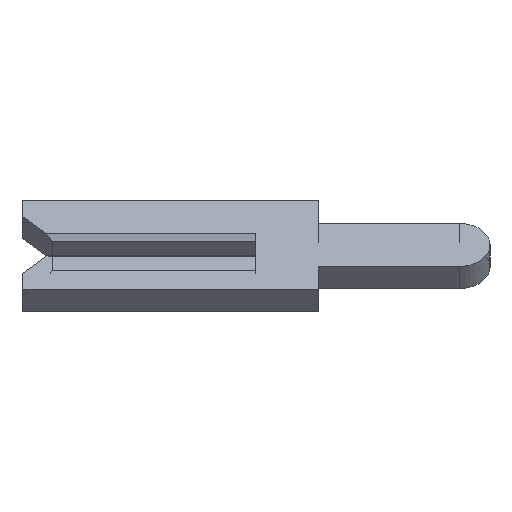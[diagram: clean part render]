
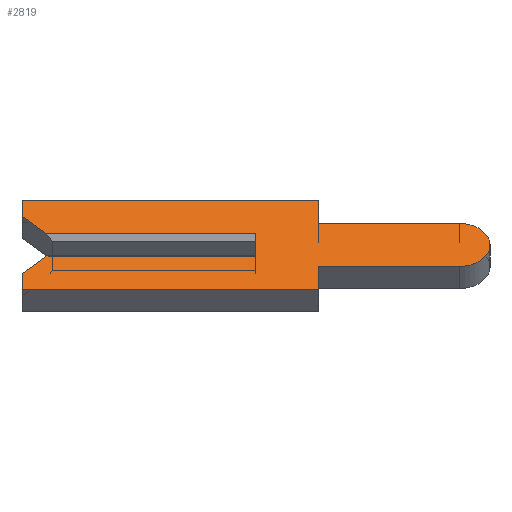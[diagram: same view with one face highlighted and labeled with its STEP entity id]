
A CAD part, left-side view. The second image highlights one B-rep face of the part: STEP entity #2819.
In plain terms, the highlighted face is planar.
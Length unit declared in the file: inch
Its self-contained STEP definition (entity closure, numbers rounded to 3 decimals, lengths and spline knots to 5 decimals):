
#10 = CARTESIAN_POINT ( 'NONE',  ( -0.01, 0.134, 0.01 ) ) ;
#25 = ORIENTED_EDGE ( 'NONE', *, *, #1651, .F. ) ;
#40 = CARTESIAN_POINT ( 'NONE',  ( -0.01, 0., -0.01 ) ) ;
#110 = CARTESIAN_POINT ( 'NONE',  ( -0.01, 0.15, 0.026 ) ) ;
#130 = CARTESIAN_POINT ( 'NONE',  ( -0.01, 0.15, -0.026 ) ) ;
#132 = FACE_OUTER_BOUND ( 'NONE', #2468, .T. ) ;
#165 = CARTESIAN_POINT ( 'NONE',  ( -0.01, 0.15, 0.01 ) ) ;
#308 = PLANE ( 'NONE',  #2267 ) ;
#331 = EDGE_CURVE ( 'NONE', #1986, #528, #2577, .T. ) ;
#369 = DIRECTION ( 'NONE',  ( 0., -1., 0. ) ) ;
#422 = VECTOR ( 'NONE', #481, 39.37008 ) ;
#441 = EDGE_CURVE ( 'NONE', #500, #1986, #459, .T. ) ;
#455 = VERTEX_POINT ( 'NONE', #2273 ) ;
#459 = LINE ( 'NONE', #110, #1696 ) ;
#465 = DIRECTION ( 'NONE',  ( 1., 0., 0. ) ) ;
#481 = DIRECTION ( 'NONE',  ( 0., 1., 0. ) ) ;
#493 = VECTOR ( 'NONE', #1460, 39.37008 ) ;
#500 = VERTEX_POINT ( 'NONE', #1653 ) ;
#506 = CARTESIAN_POINT ( 'NONE',  ( -0.01, 0.1305, -0.0065 ) ) ;
#528 = VERTEX_POINT ( 'NONE', #2779 ) ;
#538 = ORIENTED_EDGE ( 'NONE', *, *, #2256, .F. ) ;
#565 = VECTOR ( 'NONE', #2634, 39.37008 ) ;
#592 = CARTESIAN_POINT ( 'NONE',  ( -0.01, 0., 0.0065 ) ) ;
#615 = DIRECTION ( 'NONE',  ( 0., 0., -1. ) ) ;
#634 = CARTESIAN_POINT ( 'NONE',  ( -0.01, -0.04, -0.0195 ) ) ;
#653 = CARTESIAN_POINT ( 'NONE',  ( -0.01, -0.04, 0.04 ) ) ;
#698 = LINE ( 'NONE', #1627, #565 ) ;
#727 = VECTOR ( 'NONE', #1073, 39.37008 ) ;
#734 = DIRECTION ( 'NONE',  ( 0., 0., 1. ) ) ;
#789 = CARTESIAN_POINT ( 'NONE',  ( -0.01, 0., 0.01 ) ) ;
#831 = LINE ( 'NONE', #506, #1555 ) ;
#937 = VERTEX_POINT ( 'NONE', #1872 ) ;
#1053 = VECTOR ( 'NONE', #1466, 39.37008 ) ;
#1072 = EDGE_CURVE ( 'NONE', #937, #2539, #1992, .T. ) ;
#1073 = DIRECTION ( 'NONE',  ( 0., 1., 0. ) ) ;
#1092 = CARTESIAN_POINT ( 'NONE',  ( -0.01, 0.134, -0.01 ) ) ;
#1100 = CIRCLE ( 'NONE', #1520, 0.0195 ) ;
#1109 = VERTEX_POINT ( 'NONE', #2127 ) ;
#1183 = ORIENTED_EDGE ( 'NONE', *, *, #441, .F. ) ;
#1185 = CARTESIAN_POINT ( 'NONE',  ( -0.01, -0.1305, -0.0195 ) ) ;
#1255 = EDGE_CURVE ( 'NONE', #2694, #1566, #1958, .T. ) ;
#1326 = ORIENTED_EDGE ( 'NONE', *, *, #1428, .T. ) ;
#1346 = VECTOR ( 'NONE', #1954, 39.37008 ) ;
#1360 = EDGE_CURVE ( 'NONE', #1774, #2841, #2565, .T. ) ;
#1376 = DIRECTION ( 'NONE',  ( 0., -0.707, 0.707 ) ) ;
#1396 = CARTESIAN_POINT ( 'NONE',  ( -0.01, 0.15, -0.026 ) ) ;
#1405 = VECTOR ( 'NONE', #2118, 39.37008 ) ;
#1410 = DIRECTION ( 'NONE',  ( 0., 0., -1. ) ) ;
#1428 = EDGE_CURVE ( 'NONE', #2333, #1566, #2649, .T. ) ;
#1459 = LINE ( 'NONE', #1759, #1346 ) ;
#1460 = DIRECTION ( 'NONE',  ( 0., -1., 0. ) ) ;
#1466 = DIRECTION ( 'NONE',  ( 0., 0., 1. ) ) ;
#1472 = CARTESIAN_POINT ( 'NONE',  ( -0.01, -0.04, -0.04 ) ) ;
#1488 = LINE ( 'NONE', #1965, #2746 ) ;
#1520 = AXIS2_PLACEMENT_3D ( 'NONE', #2249, #465, #2211 ) ;
#1538 = DIRECTION ( 'NONE',  ( 0., 0., -1. ) ) ;
#1555 = VECTOR ( 'NONE', #1376, 39.37008 ) ;
#1566 = VERTEX_POINT ( 'NONE', #789 ) ;
#1579 = VECTOR ( 'NONE', #615, 39.37008 ) ;
#1627 = CARTESIAN_POINT ( 'NONE',  ( -0.01, 0.1305, 0.0065 ) ) ;
#1633 = ORIENTED_EDGE ( 'NONE', *, *, #1360, .F. ) ;
#1651 = EDGE_CURVE ( 'NONE', #2333, #500, #698, .T. ) ;
#1653 = CARTESIAN_POINT ( 'NONE',  ( -0.01, 0.15, 0.026 ) ) ;
#1696 = VECTOR ( 'NONE', #734, 39.37008 ) ;
#1700 = VERTEX_POINT ( 'NONE', #1092 ) ;
#1706 = EDGE_CURVE ( 'NONE', #1700, #2694, #1488, .T. ) ;
#1758 = EDGE_CURVE ( 'NONE', #2799, #1774, #2646, .T. ) ;
#1759 = CARTESIAN_POINT ( 'NONE',  ( -0.01, -0.04, 0.0195 ) ) ;
#1767 = ORIENTED_EDGE ( 'NONE', *, *, #1706, .F. ) ;
#1774 = VERTEX_POINT ( 'NONE', #2425 ) ;
#1799 = EDGE_CURVE ( 'NONE', #528, #455, #2190, .T. ) ;
#1807 = EDGE_CURVE ( 'NONE', #455, #1109, #1459, .T. ) ;
#1872 = CARTESIAN_POINT ( 'NONE',  ( -0.01, 0.15, -0.04 ) ) ;
#1954 = DIRECTION ( 'NONE',  ( 0., -1., 0. ) ) ;
#1958 = LINE ( 'NONE', #592, #1053 ) ;
#1965 = CARTESIAN_POINT ( 'NONE',  ( -0.01, -0.1305, -0.01 ) ) ;
#1986 = VERTEX_POINT ( 'NONE', #2202 ) ;
#1992 = LINE ( 'NONE', #130, #1405 ) ;
#2118 = DIRECTION ( 'NONE',  ( 0., 0., 1. ) ) ;
#2127 = CARTESIAN_POINT ( 'NONE',  ( -0.01, -0.1305, 0.0195 ) ) ;
#2152 = ORIENTED_EDGE ( 'NONE', *, *, #1072, .F. ) ;
#2154 = ORIENTED_EDGE ( 'NONE', *, *, #1807, .F. ) ;
#2166 = CARTESIAN_POINT ( 'NONE',  ( -0.01, 0.15, 0.04 ) ) ;
#2173 = DIRECTION ( 'NONE',  ( 0., -1., 0. ) ) ;
#2190 = LINE ( 'NONE', #653, #2514 ) ;
#2195 = EDGE_CURVE ( 'NONE', #1109, #2799, #1100, .T. ) ;
#2202 = CARTESIAN_POINT ( 'NONE',  ( -0.01, 0.15, 0.04 ) ) ;
#2211 = DIRECTION ( 'NONE',  ( 0., 0., -1. ) ) ;
#2222 = ORIENTED_EDGE ( 'NONE', *, *, #1758, .F. ) ;
#2234 = CARTESIAN_POINT ( 'NONE',  ( -0.01, 0.15, -0.04 ) ) ;
#2249 = CARTESIAN_POINT ( 'NONE',  ( -0.01, -0.1305, 0. ) ) ;
#2256 = EDGE_CURVE ( 'NONE', #2841, #937, #2280, .T. ) ;
#2261 = DIRECTION ( 'NONE',  ( 1., 0., 0. ) ) ;
#2267 = AXIS2_PLACEMENT_3D ( 'NONE', #2762, #2261, #1410 ) ;
#2273 = CARTESIAN_POINT ( 'NONE',  ( -0.01, -0.04, 0.0195 ) ) ;
#2280 = LINE ( 'NONE', #2234, #422 ) ;
#2333 = VERTEX_POINT ( 'NONE', #10 ) ;
#2425 = CARTESIAN_POINT ( 'NONE',  ( -0.01, -0.04, -0.0195 ) ) ;
#2468 = EDGE_LOOP ( 'NONE', ( #1326, #2472, #1767, #2729, #2152, #538, #1633, #2222, #2548, #2154, #2587, #2763, #1183, #25 ) ) ;
#2472 = ORIENTED_EDGE ( 'NONE', *, *, #1255, .F. ) ;
#2492 = CARTESIAN_POINT ( 'NONE',  ( -0.01, -0.04, -0.04 ) ) ;
#2514 = VECTOR ( 'NONE', #1538, 39.37008 ) ;
#2539 = VERTEX_POINT ( 'NONE', #1396 ) ;
#2548 = ORIENTED_EDGE ( 'NONE', *, *, #2195, .F. ) ;
#2565 = LINE ( 'NONE', #1472, #1579 ) ;
#2577 = LINE ( 'NONE', #2166, #493 ) ;
#2587 = ORIENTED_EDGE ( 'NONE', *, *, #1799, .F. ) ;
#2610 = VECTOR ( 'NONE', #369, 39.37008 ) ;
#2634 = DIRECTION ( 'NONE',  ( 0., 0.707, 0.707 ) ) ;
#2646 = LINE ( 'NONE', #634, #727 ) ;
#2649 = LINE ( 'NONE', #165, #2610 ) ;
#2694 = VERTEX_POINT ( 'NONE', #40 ) ;
#2709 = EDGE_CURVE ( 'NONE', #2539, #1700, #831, .T. ) ;
#2729 = ORIENTED_EDGE ( 'NONE', *, *, #2709, .F. ) ;
#2746 = VECTOR ( 'NONE', #2173, 39.37008 ) ;
#2762 = CARTESIAN_POINT ( 'NONE',  ( -0.01, -0.1305, 0. ) ) ;
#2763 = ORIENTED_EDGE ( 'NONE', *, *, #331, .F. ) ;
#2779 = CARTESIAN_POINT ( 'NONE',  ( -0.01, -0.04, 0.04 ) ) ;
#2799 = VERTEX_POINT ( 'NONE', #1185 ) ;
#2819 = ADVANCED_FACE ( 'NONE', ( #132 ), #308, .F. ) ;
#2841 = VERTEX_POINT ( 'NONE', #2492 ) ;
